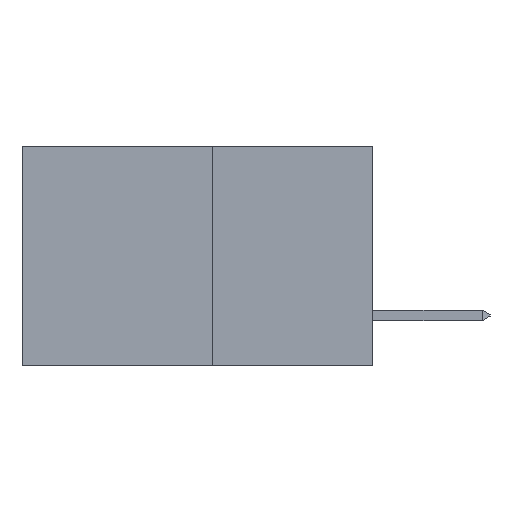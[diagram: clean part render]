
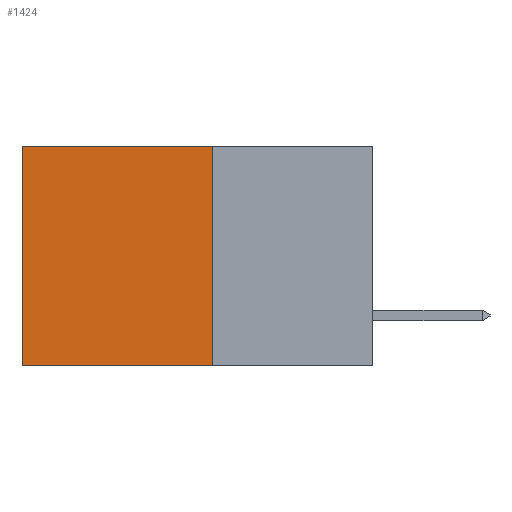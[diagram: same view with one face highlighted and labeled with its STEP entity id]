
A CAD part, left-side view. The second image highlights one B-rep face of the part: STEP entity #1424.
In plain terms, the highlighted planar face has unit normal (-1, 0, 0).
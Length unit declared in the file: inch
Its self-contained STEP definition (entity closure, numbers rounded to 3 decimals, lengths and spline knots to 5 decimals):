
#55 = DIRECTION ( 'NONE',  ( 0., 0., -1. ) ) ;
#301 = VERTEX_POINT ( 'NONE', #2886 ) ;
#481 = CARTESIAN_POINT ( 'NONE',  ( 0.277, 0.27, -0.37 ) ) ;
#809 = ORIENTED_EDGE ( 'NONE', *, *, #19162, .T. ) ;
#841 = ORIENTED_EDGE ( 'NONE', *, *, #11358, .F. ) ;
#1424 = ADVANCED_FACE ( 'NONE', ( #2755 ), #2110, .F. ) ;
#1713 = EDGE_CURVE ( 'NONE', #16504, #13682, #8699, .T. ) ;
#2100 = LINE ( 'NONE', #14373, #17157 ) ;
#2110 = PLANE ( 'NONE',  #7890 ) ;
#2755 = FACE_OUTER_BOUND ( 'NONE', #3734, .T. ) ;
#2886 = CARTESIAN_POINT ( 'NONE',  ( 0.277, 0.59, -0.37 ) ) ;
#3734 = EDGE_LOOP ( 'NONE', ( #809, #12313, #841, #17851 ) ) ;
#3804 = DIRECTION ( 'NONE',  ( 0., 0., -1. ) ) ;
#4580 = CARTESIAN_POINT ( 'NONE',  ( 0.277, 0.27, -0.37 ) ) ;
#4658 = VECTOR ( 'NONE', #15398, 39.37008 ) ;
#5512 = CARTESIAN_POINT ( 'NONE',  ( 0.277, 0.27, -0.37 ) ) ;
#7890 = AXIS2_PLACEMENT_3D ( 'NONE', #5512, #9277, #10454 ) ;
#8699 = LINE ( 'NONE', #19249, #4658 ) ;
#8775 = EDGE_CURVE ( 'NONE', #8786, #301, #18004, .T. ) ;
#8786 = VERTEX_POINT ( 'NONE', #481 ) ;
#9055 = CARTESIAN_POINT ( 'NONE',  ( 0.277, 0.59, 0. ) ) ;
#9277 = DIRECTION ( 'NONE',  ( 1., 0., 0. ) ) ;
#9583 = DIRECTION ( 'NONE',  ( 0., 1., 0. ) ) ;
#10454 = DIRECTION ( 'NONE',  ( 0., 0., -1. ) ) ;
#10858 = CARTESIAN_POINT ( 'NONE',  ( 0.277, 0.27, 0. ) ) ;
#11358 = EDGE_CURVE ( 'NONE', #16504, #8786, #19053, .T. ) ;
#12313 = ORIENTED_EDGE ( 'NONE', *, *, #8775, .F. ) ;
#13682 = VERTEX_POINT ( 'NONE', #9055 ) ;
#13699 = VECTOR ( 'NONE', #9583, 39.37008 ) ;
#14373 = CARTESIAN_POINT ( 'NONE',  ( 0.277, 0.59, -0.37 ) ) ;
#15398 = DIRECTION ( 'NONE',  ( 0., 1., 0. ) ) ;
#16504 = VERTEX_POINT ( 'NONE', #10858 ) ;
#16992 = CARTESIAN_POINT ( 'NONE',  ( 0.277, 0.27, -0.37 ) ) ;
#17157 = VECTOR ( 'NONE', #3804, 39.37008 ) ;
#17851 = ORIENTED_EDGE ( 'NONE', *, *, #1713, .T. ) ;
#18004 = LINE ( 'NONE', #16992, #13699 ) ;
#18591 = VECTOR ( 'NONE', #55, 39.37008 ) ;
#19053 = LINE ( 'NONE', #4580, #18591 ) ;
#19162 = EDGE_CURVE ( 'NONE', #13682, #301, #2100, .T. ) ;
#19249 = CARTESIAN_POINT ( 'NONE',  ( 0.277, 0.27, 0. ) ) ;
